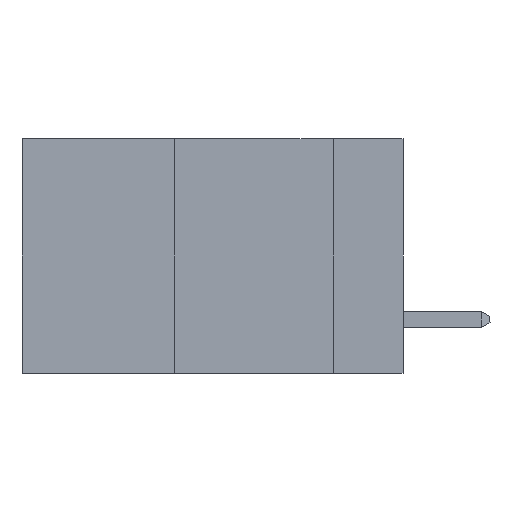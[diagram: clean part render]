
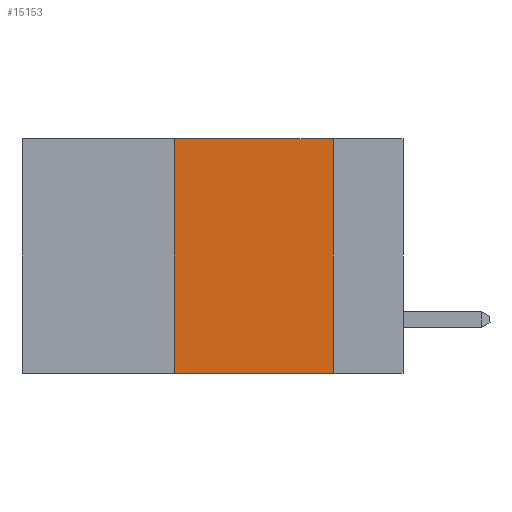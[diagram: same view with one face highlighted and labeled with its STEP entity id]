
A CAD part, left-side view. The second image highlights one B-rep face of the part: STEP entity #15153.
In plain terms, the highlighted planar face has unit normal (-1, 0, 0).
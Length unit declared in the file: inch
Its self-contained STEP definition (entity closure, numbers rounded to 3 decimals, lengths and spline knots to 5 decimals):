
#228 = VERTEX_POINT ( 'NONE', #13845 ) ;
#511 = ORIENTED_EDGE ( 'NONE', *, *, #20026, .T. ) ;
#1159 = CARTESIAN_POINT ( 'NONE',  ( 0., 0.36, 0. ) ) ;
#1190 = DIRECTION ( 'NONE',  ( 0., 0., 1. ) ) ;
#1730 = CARTESIAN_POINT ( 'NONE',  ( 0., 0.6, 0. ) ) ;
#2091 = EDGE_CURVE ( 'NONE', #4354, #7999, #4059, .T. ) ;
#2200 = ORIENTED_EDGE ( 'NONE', *, *, #13500, .F. ) ;
#2730 = CARTESIAN_POINT ( 'NONE',  ( 0., 0.6, 0. ) ) ;
#3268 = FACE_OUTER_BOUND ( 'NONE', #16629, .T. ) ;
#4059 = LINE ( 'NONE', #1159, #20765 ) ;
#4354 = VERTEX_POINT ( 'NONE', #11623 ) ;
#4415 = PLANE ( 'NONE',  #11253 ) ;
#4444 = VECTOR ( 'NONE', #20379, 39.37008 ) ;
#4483 = DIRECTION ( 'NONE',  ( 0., 0., -1. ) ) ;
#4708 = CARTESIAN_POINT ( 'NONE',  ( 0., 0.36, 0. ) ) ;
#6377 = ORIENTED_EDGE ( 'NONE', *, *, #15432, .F. ) ;
#7999 = VERTEX_POINT ( 'NONE', #4708 ) ;
#8666 = DIRECTION ( 'NONE',  ( 0., -1., 0. ) ) ;
#9642 = VECTOR ( 'NONE', #13976, 39.37008 ) ;
#11253 = AXIS2_PLACEMENT_3D ( 'NONE', #2730, #14546, #4483 ) ;
#11623 = CARTESIAN_POINT ( 'NONE',  ( 0., 0.36, -0.37 ) ) ;
#13500 = EDGE_CURVE ( 'NONE', #228, #20974, #17554, .T. ) ;
#13845 = CARTESIAN_POINT ( 'NONE',  ( 0., 0.11, 0. ) ) ;
#13976 = DIRECTION ( 'NONE',  ( 0., -1., 0. ) ) ;
#14033 = LINE ( 'NONE', #15476, #9642 ) ;
#14546 = DIRECTION ( 'NONE',  ( 1., 0., 0. ) ) ;
#14835 = LINE ( 'NONE', #1730, #18846 ) ;
#15153 = ADVANCED_FACE ( 'NONE', ( #3268 ), #4415, .F. ) ;
#15432 = EDGE_CURVE ( 'NONE', #7999, #228, #14835, .T. ) ;
#15476 = CARTESIAN_POINT ( 'NONE',  ( 0., 0.6, -0.37 ) ) ;
#15872 = ORIENTED_EDGE ( 'NONE', *, *, #2091, .F. ) ;
#16629 = EDGE_LOOP ( 'NONE', ( #2200, #6377, #15872, #511 ) ) ;
#17554 = LINE ( 'NONE', #18847, #4444 ) ;
#18846 = VECTOR ( 'NONE', #8666, 39.37008 ) ;
#18847 = CARTESIAN_POINT ( 'NONE',  ( 0., 0.11, 0. ) ) ;
#20026 = EDGE_CURVE ( 'NONE', #4354, #20974, #14033, .T. ) ;
#20379 = DIRECTION ( 'NONE',  ( 0., 0., -1. ) ) ;
#20765 = VECTOR ( 'NONE', #1190, 39.37008 ) ;
#20864 = CARTESIAN_POINT ( 'NONE',  ( 0., 0.11, -0.37 ) ) ;
#20974 = VERTEX_POINT ( 'NONE', #20864 ) ;
